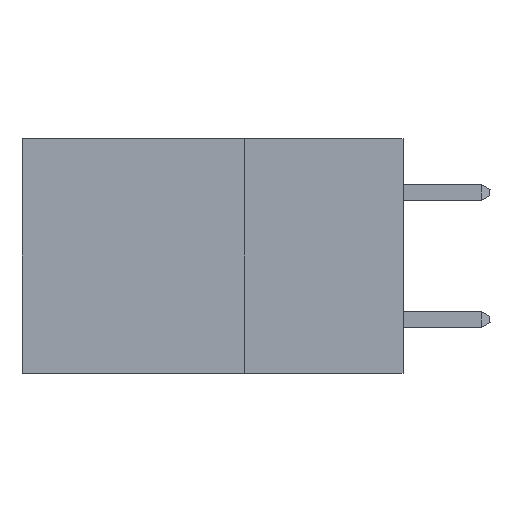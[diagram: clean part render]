
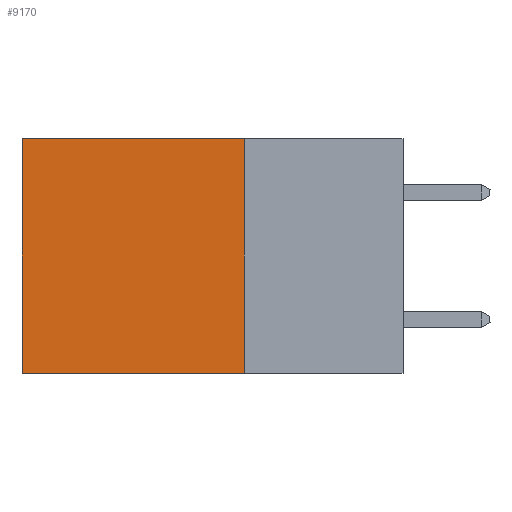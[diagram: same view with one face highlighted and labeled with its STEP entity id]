
A CAD part, left-side view. The second image highlights one B-rep face of the part: STEP entity #9170.
In plain terms, the highlighted planar face has unit normal (-1, 0, 0).
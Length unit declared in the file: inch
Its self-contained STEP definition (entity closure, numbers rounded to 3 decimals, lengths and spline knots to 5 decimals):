
#55 = CARTESIAN_POINT ( 'NONE',  ( 0.2875, 0.25, 0. ) ) ;
#198 = VERTEX_POINT ( 'NONE', #329 ) ;
#329 = CARTESIAN_POINT ( 'NONE',  ( 0.2875, 0.25, -0.37 ) ) ;
#2549 = CARTESIAN_POINT ( 'NONE',  ( 0.2875, 0.6, -0.37 ) ) ;
#2560 = EDGE_CURVE ( 'NONE', #31186, #198, #32433, .T. ) ;
#2598 = DIRECTION ( 'NONE',  ( 0., 0., -1. ) ) ;
#2845 = LINE ( 'NONE', #55, #19148 ) ;
#3305 = VERTEX_POINT ( 'NONE', #2549 ) ;
#3377 = CARTESIAN_POINT ( 'NONE',  ( 0.2875, 0.25, 0. ) ) ;
#4456 = CARTESIAN_POINT ( 'NONE',  ( 0.2875, 0.6, 0. ) ) ;
#4560 = VECTOR ( 'NONE', #21560, 39.37008 ) ;
#4822 = DIRECTION ( 'NONE',  ( 1., 0., 0. ) ) ;
#5122 = ORIENTED_EDGE ( 'NONE', *, *, #21919, .F. ) ;
#9170 = ADVANCED_FACE ( 'NONE', ( #19575 ), #20272, .F. ) ;
#13122 = ORIENTED_EDGE ( 'NONE', *, *, #24821, .T. ) ;
#13637 = ORIENTED_EDGE ( 'NONE', *, *, #2560, .F. ) ;
#14680 = LINE ( 'NONE', #4456, #26184 ) ;
#18164 = VECTOR ( 'NONE', #18731, 39.37008 ) ;
#18731 = DIRECTION ( 'NONE',  ( 0., 0., -1. ) ) ;
#19148 = VECTOR ( 'NONE', #20392, 39.37008 ) ;
#19575 = FACE_OUTER_BOUND ( 'NONE', #31430, .T. ) ;
#20272 = PLANE ( 'NONE',  #28565 ) ;
#20392 = DIRECTION ( 'NONE',  ( 0., 1., 0. ) ) ;
#21560 = DIRECTION ( 'NONE',  ( 0., 1., 0. ) ) ;
#21919 = EDGE_CURVE ( 'NONE', #198, #3305, #22846, .T. ) ;
#22632 = CARTESIAN_POINT ( 'NONE',  ( 0.2875, 0.6, 0. ) ) ;
#22846 = LINE ( 'NONE', #32208, #4560 ) ;
#24821 = EDGE_CURVE ( 'NONE', #31186, #29710, #2845, .T. ) ;
#26184 = VECTOR ( 'NONE', #27329, 39.37008 ) ;
#26523 = EDGE_CURVE ( 'NONE', #29710, #3305, #14680, .T. ) ;
#27329 = DIRECTION ( 'NONE',  ( 0., 0., -1. ) ) ;
#28565 = AXIS2_PLACEMENT_3D ( 'NONE', #30037, #4822, #2598 ) ;
#28893 = CARTESIAN_POINT ( 'NONE',  ( 0.2875, 0.25, 0. ) ) ;
#29710 = VERTEX_POINT ( 'NONE', #22632 ) ;
#30037 = CARTESIAN_POINT ( 'NONE',  ( 0.2875, 0.25, 0. ) ) ;
#31186 = VERTEX_POINT ( 'NONE', #28893 ) ;
#31430 = EDGE_LOOP ( 'NONE', ( #31803, #5122, #13637, #13122 ) ) ;
#31803 = ORIENTED_EDGE ( 'NONE', *, *, #26523, .T. ) ;
#32208 = CARTESIAN_POINT ( 'NONE',  ( 0.2875, 0.25, -0.37 ) ) ;
#32433 = LINE ( 'NONE', #3377, #18164 ) ;
